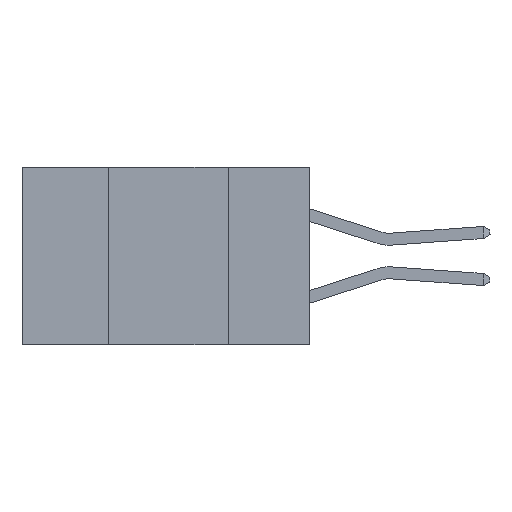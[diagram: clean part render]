
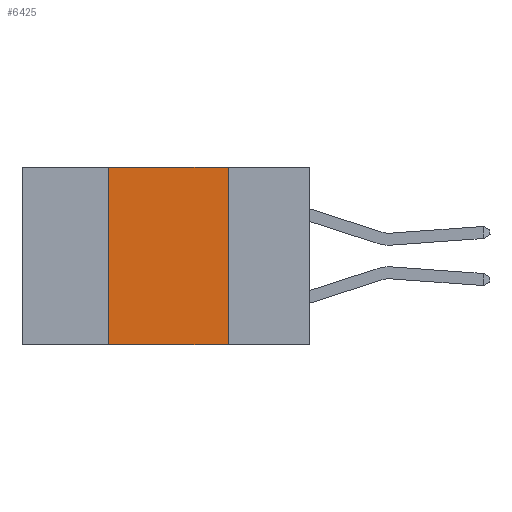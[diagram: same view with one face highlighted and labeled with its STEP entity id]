
A CAD part, left-side view. The second image highlights one B-rep face of the part: STEP entity #6425.
In plain terms, the highlighted planar face has unit normal (-1, 0, 0).
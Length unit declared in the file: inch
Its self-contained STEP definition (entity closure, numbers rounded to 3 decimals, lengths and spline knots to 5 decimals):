
#792 = ORIENTED_EDGE ( 'NONE', *, *, #8710, .F. ) ;
#849 = CARTESIAN_POINT ( 'NONE',  ( 0., 0.6, -0.37 ) ) ;
#897 = VECTOR ( 'NONE', #1174, 39.37008 ) ;
#1094 = CARTESIAN_POINT ( 'NONE',  ( 0., 0.17, -0.37 ) ) ;
#1174 = DIRECTION ( 'NONE',  ( 0., 0., -1. ) ) ;
#1306 = EDGE_CURVE ( 'NONE', #4694, #2985, #4105, .T. ) ;
#1392 = DIRECTION ( 'NONE',  ( 0., 0., -1. ) ) ;
#1441 = CARTESIAN_POINT ( 'NONE',  ( 0., 0.42, -0.37 ) ) ;
#1588 = CARTESIAN_POINT ( 'NONE',  ( 0., 0.6, 0. ) ) ;
#1627 = VERTEX_POINT ( 'NONE', #1441 ) ;
#1667 = DIRECTION ( 'NONE',  ( 0., -1., 0. ) ) ;
#2028 = VERTEX_POINT ( 'NONE', #8155 ) ;
#2214 = PLANE ( 'NONE',  #3932 ) ;
#2233 = CARTESIAN_POINT ( 'NONE',  ( 0., 0.6, 0. ) ) ;
#2512 = DIRECTION ( 'NONE',  ( 0., 0., 1. ) ) ;
#2608 = LINE ( 'NONE', #1094, #897 ) ;
#2730 = VECTOR ( 'NONE', #7610, 39.37008 ) ;
#2792 = DIRECTION ( 'NONE',  ( 1., 0., 0. ) ) ;
#2985 = VERTEX_POINT ( 'NONE', #7248 ) ;
#3195 = VECTOR ( 'NONE', #1667, 39.37008 ) ;
#3309 = ORIENTED_EDGE ( 'NONE', *, *, #1306, .F. ) ;
#3932 = AXIS2_PLACEMENT_3D ( 'NONE', #1588, #2792, #1392 ) ;
#4105 = LINE ( 'NONE', #2233, #2730 ) ;
#4518 = VECTOR ( 'NONE', #2512, 39.37008 ) ;
#4694 = VERTEX_POINT ( 'NONE', #4874 ) ;
#4874 = CARTESIAN_POINT ( 'NONE',  ( 0., 0.42, 0. ) ) ;
#4951 = FACE_OUTER_BOUND ( 'NONE', #6354, .T. ) ;
#5044 = LINE ( 'NONE', #849, #3195 ) ;
#5093 = EDGE_CURVE ( 'NONE', #2985, #2028, #2608, .T. ) ;
#5750 = EDGE_CURVE ( 'NONE', #1627, #2028, #5044, .T. ) ;
#5947 = CARTESIAN_POINT ( 'NONE',  ( 0., 0.42, -0.37 ) ) ;
#6354 = EDGE_LOOP ( 'NONE', ( #7465, #3309, #792, #7269 ) ) ;
#6425 = ADVANCED_FACE ( 'NONE', ( #4951 ), #2214, .F. ) ;
#7248 = CARTESIAN_POINT ( 'NONE',  ( 0., 0.17, 0. ) ) ;
#7269 = ORIENTED_EDGE ( 'NONE', *, *, #5750, .T. ) ;
#7465 = ORIENTED_EDGE ( 'NONE', *, *, #5093, .F. ) ;
#7610 = DIRECTION ( 'NONE',  ( 0., -1., 0. ) ) ;
#8155 = CARTESIAN_POINT ( 'NONE',  ( 0., 0.17, -0.37 ) ) ;
#8557 = LINE ( 'NONE', #5947, #4518 ) ;
#8710 = EDGE_CURVE ( 'NONE', #1627, #4694, #8557, .T. ) ;
